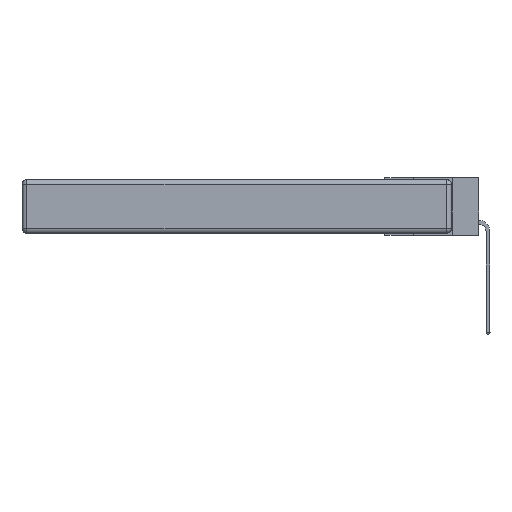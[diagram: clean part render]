
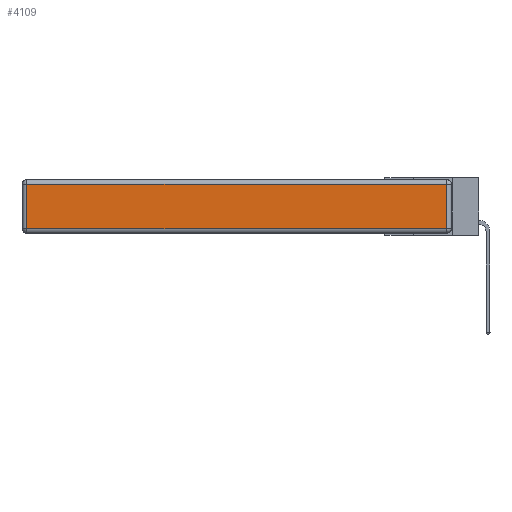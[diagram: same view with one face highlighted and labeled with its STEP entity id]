
A CAD part, left-side view. The second image highlights one B-rep face of the part: STEP entity #4109.
In plain terms, the highlighted planar face has unit normal (-1, 0, 0).
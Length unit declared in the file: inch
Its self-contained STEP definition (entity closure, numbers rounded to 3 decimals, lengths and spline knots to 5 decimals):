
#86 = LINE ( 'NONE', #1924, #8474 ) ;
#281 = PLANE ( 'NONE',  #11918 ) ;
#783 = EDGE_CURVE ( 'NONE', #13770, #11727, #7798, .T. ) ;
#1015 = VECTOR ( 'NONE', #8759, 39.37008 ) ;
#1417 = VECTOR ( 'NONE', #18629, 39.37008 ) ;
#1924 = CARTESIAN_POINT ( 'NONE',  ( 0., 0., -0.313 ) ) ;
#2811 = CARTESIAN_POINT ( 'NONE',  ( 0., 2.75, -0.03 ) ) ;
#3323 = EDGE_CURVE ( 'NONE', #8673, #13770, #21272, .T. ) ;
#3564 = DIRECTION ( 'NONE',  ( 0., -1., 0. ) ) ;
#4109 = ADVANCED_FACE ( 'NONE', ( #7530 ), #281, .T. ) ;
#4930 = VERTEX_POINT ( 'NONE', #5046 ) ;
#5046 = CARTESIAN_POINT ( 'NONE',  ( 0., 2.72, -0.313 ) ) ;
#6393 = DIRECTION ( 'NONE',  ( 0., 1., 0. ) ) ;
#6873 = ORIENTED_EDGE ( 'NONE', *, *, #7517, .T. ) ;
#6909 = EDGE_CURVE ( 'NONE', #4930, #8673, #86, .T. ) ;
#7517 = EDGE_CURVE ( 'NONE', #11727, #4930, #21706, .T. ) ;
#7530 = FACE_OUTER_BOUND ( 'NONE', #20280, .T. ) ;
#7798 = LINE ( 'NONE', #2811, #10875 ) ;
#8474 = VECTOR ( 'NONE', #3564, 39.37008 ) ;
#8673 = VERTEX_POINT ( 'NONE', #14064 ) ;
#8759 = DIRECTION ( 'NONE',  ( 0., 0., -1. ) ) ;
#10591 = ORIENTED_EDGE ( 'NONE', *, *, #3323, .T. ) ;
#10875 = VECTOR ( 'NONE', #6393, 39.37008 ) ;
#11564 = CARTESIAN_POINT ( 'NONE',  ( 0., 0.03, -0.343 ) ) ;
#11727 = VERTEX_POINT ( 'NONE', #19323 ) ;
#11918 = AXIS2_PLACEMENT_3D ( 'NONE', #19967, #16315, #21899 ) ;
#12492 = ORIENTED_EDGE ( 'NONE', *, *, #783, .T. ) ;
#13770 = VERTEX_POINT ( 'NONE', #16106 ) ;
#14004 = CARTESIAN_POINT ( 'NONE',  ( 0., 2.72, -0.343 ) ) ;
#14064 = CARTESIAN_POINT ( 'NONE',  ( 0., 0.03, -0.313 ) ) ;
#16106 = CARTESIAN_POINT ( 'NONE',  ( 0., 0.03, -0.03 ) ) ;
#16315 = DIRECTION ( 'NONE',  ( -1., 0., 0. ) ) ;
#18320 = ORIENTED_EDGE ( 'NONE', *, *, #6909, .T. ) ;
#18629 = DIRECTION ( 'NONE',  ( 0., 0., 1. ) ) ;
#19323 = CARTESIAN_POINT ( 'NONE',  ( 0., 2.72, -0.03 ) ) ;
#19967 = CARTESIAN_POINT ( 'NONE',  ( 0., 0., -0.343 ) ) ;
#20280 = EDGE_LOOP ( 'NONE', ( #18320, #10591, #12492, #6873 ) ) ;
#21272 = LINE ( 'NONE', #11564, #1417 ) ;
#21706 = LINE ( 'NONE', #14004, #1015 ) ;
#21899 = DIRECTION ( 'NONE',  ( 0., 0., 1. ) ) ;
